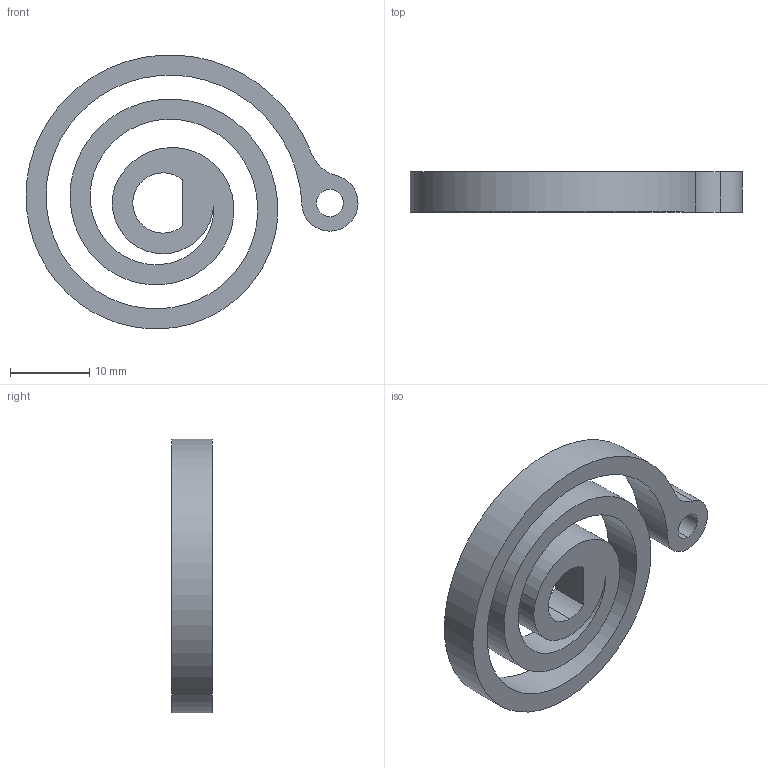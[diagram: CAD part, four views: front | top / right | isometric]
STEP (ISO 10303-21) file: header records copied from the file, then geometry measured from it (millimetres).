
FILE_DESCRIPTION (( 'STEP AP214' ), '1' );
FILE_NAME ('coilspringX2.STEP', '2013-10-27T06:43:03', ( 'Matt' ), ( '' ), 'SwSTEP 2.0', 'SolidWorks 2013', '' );
FILE_SCHEMA (( 'AUTOMOTIVE_DESIGN' ));
Length unit declared in the file: inch
Products named in the file (1): coilspringX2
Bounding box: 41.93 x 5.08 x 34.55 mm (x, y, z)
Volume: 2825.2 mm3; surface area: 3260.7 mm2
Topology: 1 solids, 1 shells, 16 faces, 42 edges, 28 vertices
Faces by surface type: cylinder 10, bspline 3, plane 3
Entity records: 996 total; most frequent: CARTESIAN_POINT 550, ORIENTED_EDGE 84, DIRECTION 84, EDGE_CURVE 42, AXIS2_PLACEMENT_3D 34, VERTEX_POINT 28, EDGE_LOOP 20, CIRCLE 20
